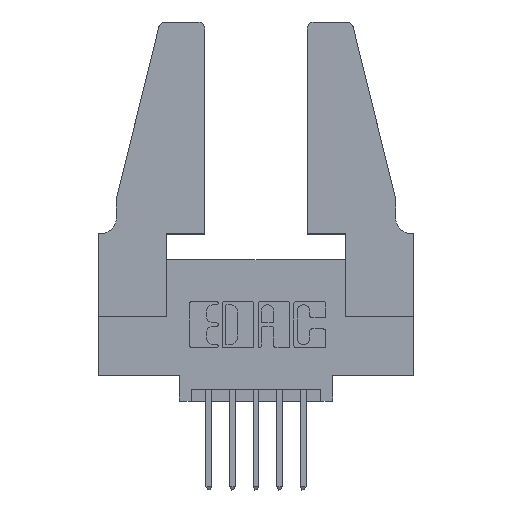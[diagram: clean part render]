
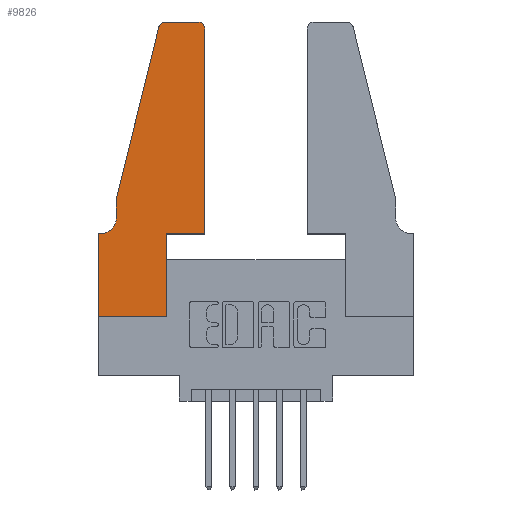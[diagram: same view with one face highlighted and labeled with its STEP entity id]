
A CAD part, top view. The second image highlights one B-rep face of the part: STEP entity #9826.
In plain terms, the highlighted planar face has unit normal (0, 0, 1).
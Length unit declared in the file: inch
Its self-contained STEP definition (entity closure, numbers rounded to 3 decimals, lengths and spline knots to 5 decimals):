
#14 = CARTESIAN_POINT ( 'NONE',  ( 0.2865, 0.35, 0.37 ) ) ;
#105 = DIRECTION ( 'NONE',  ( 0., 0., 1. ) ) ;
#325 = ORIENTED_EDGE ( 'NONE', *, *, #1920, .T. ) ;
#487 = DIRECTION ( 'NONE',  ( 0., 0., -1. ) ) ;
#621 = VECTOR ( 'NONE', #8792, 39.37008 ) ;
#855 = CARTESIAN_POINT ( 'NONE',  ( 0.2605, 1.25, 0.37 ) ) ;
#916 = CARTESIAN_POINT ( 'NONE',  ( 0.4505, 0.35, 0.37 ) ) ;
#1222 = VERTEX_POINT ( 'NONE', #8852 ) ;
#1288 = VECTOR ( 'NONE', #9902, 39.37008 ) ;
#1628 = DIRECTION ( 'NONE',  ( 0., 0., 1. ) ) ;
#1654 = ORIENTED_EDGE ( 'NONE', *, *, #6025, .T. ) ;
#1756 = ORIENTED_EDGE ( 'NONE', *, *, #3448, .T. ) ;
#1772 = LINE ( 'NONE', #3541, #6079 ) ;
#1785 = VECTOR ( 'NONE', #9576, 39.37008 ) ;
#1920 = EDGE_CURVE ( 'NONE', #7759, #7304, #6162, .T. ) ;
#2629 = VERTEX_POINT ( 'NONE', #10816 ) ;
#2794 = EDGE_CURVE ( 'NONE', #10109, #5628, #11188, .T. ) ;
#2859 = CARTESIAN_POINT ( 'NONE',  ( 0., 0.35, 0.37 ) ) ;
#2902 = CARTESIAN_POINT ( 'NONE',  ( 0.4205, 1.22, 0.37 ) ) ;
#2922 = CARTESIAN_POINT ( 'NONE',  ( 0.25487, 1.22718, 0.37 ) ) ;
#3305 = CARTESIAN_POINT ( 'NONE',  ( 0.0755, 0.5, 0.37 ) ) ;
#3308 = DIRECTION ( 'NONE',  ( -1., 0., 0. ) ) ;
#3335 = CIRCLE ( 'NONE', #8166, 0.03 ) ;
#3448 = EDGE_CURVE ( 'NONE', #8678, #7759, #8823, .T. ) ;
#3493 = CARTESIAN_POINT ( 'NONE',  ( 0.4505, 0.35, 0.37 ) ) ;
#3541 = CARTESIAN_POINT ( 'NONE',  ( 0.4505, 0.35, 0.37 ) ) ;
#3762 = DIRECTION ( 'NONE',  ( 1., 0., 0. ) ) ;
#3815 = EDGE_CURVE ( 'NONE', #5628, #2629, #5324, .T. ) ;
#3831 = CIRCLE ( 'NONE', #9519, 0.03 ) ;
#3854 = EDGE_CURVE ( 'NONE', #4739, #9630, #3335, .T. ) ;
#3873 = LINE ( 'NONE', #4981, #5842 ) ;
#4097 = LINE ( 'NONE', #855, #6356 ) ;
#4182 = VERTEX_POINT ( 'NONE', #10939 ) ;
#4289 = VECTOR ( 'NONE', #7004, 39.37008 ) ;
#4379 = DIRECTION ( 'NONE',  ( 0., -1., 0. ) ) ;
#4383 = CARTESIAN_POINT ( 'NONE',  ( 0., 0., 0.37 ) ) ;
#4529 = VECTOR ( 'NONE', #10762, 39.37008 ) ;
#4728 = ORIENTED_EDGE ( 'NONE', *, *, #10423, .T. ) ;
#4739 = VERTEX_POINT ( 'NONE', #5063 ) ;
#4751 = ORIENTED_EDGE ( 'NONE', *, *, #3854, .T. ) ;
#4924 = CARTESIAN_POINT ( 'NONE',  ( 0., 0.35, 0.37 ) ) ;
#4981 = CARTESIAN_POINT ( 'NONE',  ( 0.0755, 0.35, 0.37 ) ) ;
#5063 = CARTESIAN_POINT ( 'NONE',  ( 0.4505, 1.22, 0.37 ) ) ;
#5194 = ORIENTED_EDGE ( 'NONE', *, *, #7994, .T. ) ;
#5324 = LINE ( 'NONE', #8749, #621 ) ;
#5418 = PLANE ( 'NONE',  #5655 ) ;
#5447 = VERTEX_POINT ( 'NONE', #3493 ) ;
#5476 = EDGE_CURVE ( 'NONE', #9630, #10776, #4097, .T. ) ;
#5628 = VERTEX_POINT ( 'NONE', #8835 ) ;
#5655 = AXIS2_PLACEMENT_3D ( 'NONE', #2859, #105, #6270 ) ;
#5769 = CARTESIAN_POINT ( 'NONE',  ( 0.0055, 0.42, 0.37 ) ) ;
#5842 = VECTOR ( 'NONE', #3308, 39.37008 ) ;
#6000 = ORIENTED_EDGE ( 'NONE', *, *, #10722, .T. ) ;
#6025 = EDGE_CURVE ( 'NONE', #10776, #8678, #3831, .T. ) ;
#6079 = VECTOR ( 'NONE', #8650, 39.37008 ) ;
#6086 = DIRECTION ( 'NONE',  ( -1., 0., 0. ) ) ;
#6162 = LINE ( 'NONE', #10610, #1288 ) ;
#6270 = DIRECTION ( 'NONE',  ( 1., 0., 0. ) ) ;
#6356 = VECTOR ( 'NONE', #6086, 39.37008 ) ;
#6623 = DIRECTION ( 'NONE',  ( -1., 0., 0. ) ) ;
#6677 = VECTOR ( 'NONE', #4379, 39.37008 ) ;
#6757 = CARTESIAN_POINT ( 'NONE',  ( 0.4205, 1.25, 0.37 ) ) ;
#6787 = CARTESIAN_POINT ( 'NONE',  ( 0.284, 1.22, 0.37 ) ) ;
#7004 = DIRECTION ( 'NONE',  ( 0., 1., 0. ) ) ;
#7070 = ORIENTED_EDGE ( 'NONE', *, *, #5476, .T. ) ;
#7304 = VERTEX_POINT ( 'NONE', #8716 ) ;
#7656 = DIRECTION ( 'NONE',  ( 1., 0., 0. ) ) ;
#7759 = VERTEX_POINT ( 'NONE', #3305 ) ;
#7870 = ORIENTED_EDGE ( 'NONE', *, *, #2794, .T. ) ;
#7994 = EDGE_CURVE ( 'NONE', #5447, #4739, #10797, .T. ) ;
#8142 = CARTESIAN_POINT ( 'NONE',  ( 0.0755, 0.5, 0.37 ) ) ;
#8166 = AXIS2_PLACEMENT_3D ( 'NONE', #2902, #8868, #3762 ) ;
#8170 = ORIENTED_EDGE ( 'NONE', *, *, #10871, .T. ) ;
#8611 = AXIS2_PLACEMENT_3D ( 'NONE', #5769, #487, #6623 ) ;
#8650 = DIRECTION ( 'NONE',  ( 1., 0., 0. ) ) ;
#8678 = VERTEX_POINT ( 'NONE', #2922 ) ;
#8716 = CARTESIAN_POINT ( 'NONE',  ( 0.0755, 0.42, 0.37 ) ) ;
#8749 = CARTESIAN_POINT ( 'NONE',  ( 0., 0., 0.37 ) ) ;
#8754 = ORIENTED_EDGE ( 'NONE', *, *, #9575, .T. ) ;
#8792 = DIRECTION ( 'NONE',  ( 1., 0., 0. ) ) ;
#8823 = LINE ( 'NONE', #8142, #4529 ) ;
#8835 = CARTESIAN_POINT ( 'NONE',  ( 0., 0., 0.37 ) ) ;
#8852 = CARTESIAN_POINT ( 'NONE',  ( 0.2865, 0.35, 0.37 ) ) ;
#8868 = DIRECTION ( 'NONE',  ( 0., 0., 1. ) ) ;
#9198 = CARTESIAN_POINT ( 'NONE',  ( 0.284, 1.25, 0.37 ) ) ;
#9224 = ORIENTED_EDGE ( 'NONE', *, *, #3815, .T. ) ;
#9519 = AXIS2_PLACEMENT_3D ( 'NONE', #6787, #1628, #7656 ) ;
#9575 = EDGE_CURVE ( 'NONE', #4182, #10109, #3873, .T. ) ;
#9576 = DIRECTION ( 'NONE',  ( 0., 1., 0. ) ) ;
#9630 = VERTEX_POINT ( 'NONE', #6757 ) ;
#9826 = ADVANCED_FACE ( 'NONE', ( #10483 ), #5418, .T. ) ;
#9902 = DIRECTION ( 'NONE',  ( 0., -1., 0. ) ) ;
#9945 = CIRCLE ( 'NONE', #8611, 0.07 ) ;
#10109 = VERTEX_POINT ( 'NONE', #4924 ) ;
#10423 = EDGE_CURVE ( 'NONE', #2629, #1222, #10601, .T. ) ;
#10483 = FACE_OUTER_BOUND ( 'NONE', #10928, .T. ) ;
#10601 = LINE ( 'NONE', #14, #1785 ) ;
#10610 = CARTESIAN_POINT ( 'NONE',  ( 0.0755, 0.5, 0.37 ) ) ;
#10722 = EDGE_CURVE ( 'NONE', #7304, #4182, #9945, .T. ) ;
#10762 = DIRECTION ( 'NONE',  ( -0.239, -0.971, 0. ) ) ;
#10776 = VERTEX_POINT ( 'NONE', #9198 ) ;
#10797 = LINE ( 'NONE', #916, #4289 ) ;
#10816 = CARTESIAN_POINT ( 'NONE',  ( 0.2865, 0., 0.37 ) ) ;
#10871 = EDGE_CURVE ( 'NONE', #1222, #5447, #1772, .T. ) ;
#10928 = EDGE_LOOP ( 'NONE', ( #7070, #1654, #1756, #325, #6000, #8754, #7870, #9224, #4728, #8170, #5194, #4751 ) ) ;
#10939 = CARTESIAN_POINT ( 'NONE',  ( 0.0055, 0.35, 0.37 ) ) ;
#11188 = LINE ( 'NONE', #4383, #6677 ) ;
